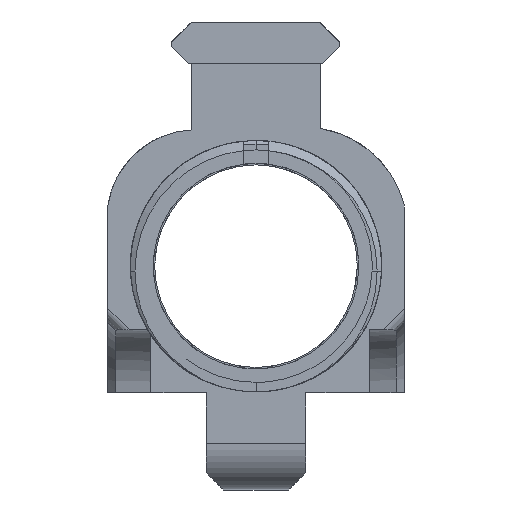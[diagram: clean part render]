
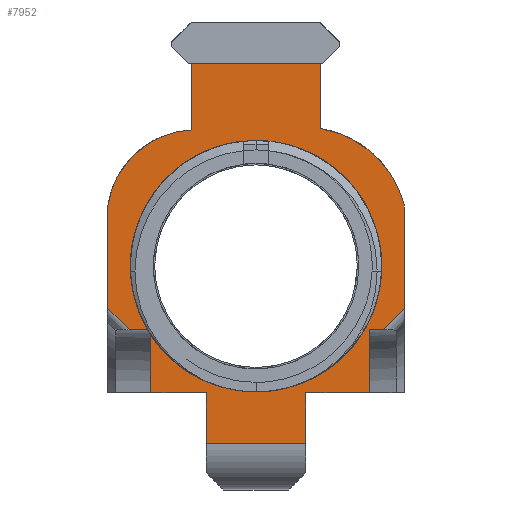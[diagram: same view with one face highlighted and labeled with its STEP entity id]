
A CAD part, front view. The second image highlights one B-rep face of the part: STEP entity #7952.
In plain terms, the highlighted planar face has unit normal (0, -1, 0).
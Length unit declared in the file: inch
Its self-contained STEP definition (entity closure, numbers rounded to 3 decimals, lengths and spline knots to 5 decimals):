
#28=FACE_BOUND('',#1369,.T.);
#355=PLANE('',#8558);
#369=CIRCLE('',#7998,0.51729);
#529=CIRCLE('',#8515,0.44384);
#537=CIRCLE('',#8557,0.58625);
#949=FACE_OUTER_BOUND('',#1368,.T.);
#1368=EDGE_LOOP('',(#7317,#7318,#7319,#7320,#7321,#7322,#7323,#7324,#7325,
#7326,#7327,#7328,#7329,#7330,#7331,#7332,#7333,#7334,#7335,#7336));
#1369=EDGE_LOOP('',(#7337));
#1472=B_SPLINE_CURVE_WITH_KNOTS('',3,(#12168,#12169,#12170,#12171),
 .UNSPECIFIED.,.F.,.F.,(4,4),(0.18081,0.55432),
 .UNSPECIFIED.);
#1555=B_SPLINE_CURVE_WITH_KNOTS('',3,(#15086,#15087,#15088,#15089),
 .UNSPECIFIED.,.F.,.F.,(4,4),(2.0691,2.45646),
 .UNSPECIFIED.);
#1620=LINE('',#11397,#2382);
#1637=LINE('',#11438,#2399);
#1769=LINE('',#12685,#2531);
#1799=LINE('',#12870,#2561);
#1881=LINE('',#13045,#2643);
#2091=LINE('',#13915,#2853);
#2271=LINE('',#14954,#3033);
#2273=LINE('',#14959,#3035);
#2275=LINE('',#14965,#3037);
#2277=LINE('',#14969,#3039);
#2283=LINE('',#14992,#3045);
#2284=LINE('',#14994,#3046);
#2290=LINE('',#15031,#3052);
#2327=LINE('',#15381,#3089);
#2358=LINE('',#16108,#3120);
#2359=LINE('',#16109,#3121);
#2382=VECTOR('',#8627,0.3937);
#2399=VECTOR('',#8654,0.3937);
#2531=VECTOR('',#8962,0.3937);
#2561=VECTOR('',#9072,0.3937);
#2643=VECTOR('',#9180,0.3937);
#2853=VECTOR('',#9658,0.494);
#3033=VECTOR('',#10202,0.3937);
#3035=VECTOR('',#10208,0.3937);
#3037=VECTOR('',#10214,0.3937);
#3039=VECTOR('',#10218,0.3937);
#3045=VECTOR('',#10234,0.3937);
#3046=VECTOR('',#10235,0.3937);
#3052=VECTOR('',#10243,0.3937);
#3089=VECTOR('',#10352,0.3937);
#3120=VECTOR('',#10473,0.3937);
#3121=VECTOR('',#10474,0.3937);
#3175=VERTEX_POINT('',#11289);
#3176=VERTEX_POINT('',#11291);
#3183=VERTEX_POINT('',#11396);
#3202=VERTEX_POINT('',#11436);
#3354=VERTEX_POINT('',#12156);
#3355=VERTEX_POINT('',#12167);
#3388=VERTEX_POINT('',#12683);
#3389=VERTEX_POINT('',#12684);
#3441=VERTEX_POINT('',#12868);
#3442=VERTEX_POINT('',#12869);
#3521=VERTEX_POINT('',#13043);
#3522=VERTEX_POINT('',#13044);
#3810=VERTEX_POINT('',#14958);
#3812=VERTEX_POINT('',#14964);
#3813=VERTEX_POINT('',#14968);
#3822=VERTEX_POINT('',#14993);
#3829=VERTEX_POINT('',#15030);
#3832=VERTEX_POINT('',#15062);
#3833=VERTEX_POINT('',#15073);
#3877=VERTEX_POINT('',#15380);
#3908=VERTEX_POINT('',#16104);
#3959=EDGE_CURVE('',#3176,#3175,#369,.T.);
#3971=EDGE_CURVE('',#3183,#3176,#1620,.T.);
#3992=EDGE_CURVE('',#3175,#3202,#1637,.F.);
#4174=EDGE_CURVE('',#3354,#3355,#1472,.T.);
#4216=EDGE_CURVE('',#3388,#3389,#1769,.F.);
#4281=EDGE_CURVE('',#3441,#3442,#1799,.T.);
#4369=EDGE_CURVE('',#3521,#3522,#1881,.F.);
#4627=EDGE_CURVE('',#3389,#3521,#2091,.T.);
#4901=EDGE_CURVE('',#3354,#3183,#2271,.T.);
#4904=EDGE_CURVE('',#3810,#3355,#2273,.T.);
#4907=EDGE_CURVE('',#3812,#3810,#2275,.T.);
#4909=EDGE_CURVE('',#3813,#3812,#2277,.T.);
#4920=EDGE_CURVE('',#3813,#3522,#2283,.T.);
#4921=EDGE_CURVE('',#3388,#3822,#2284,.T.);
#4930=EDGE_CURVE('',#3829,#3822,#2290,.T.);
#4937=EDGE_CURVE('',#3833,#3832,#1555,.T.);
#5005=EDGE_CURVE('',#3832,#3877,#2327,.T.);
#5010=EDGE_CURVE('',#3441,#3877,#529,.T.);
#5083=EDGE_CURVE('',#3908,#3908,#537,.T.);
#5084=EDGE_CURVE('',#3202,#3442,#2358,.T.);
#5085=EDGE_CURVE('',#3833,#3829,#2359,.T.);
#7317=ORIENTED_EDGE('',*,*,#5084,.T.);
#7318=ORIENTED_EDGE('',*,*,#4281,.F.);
#7319=ORIENTED_EDGE('',*,*,#5010,.T.);
#7320=ORIENTED_EDGE('',*,*,#5005,.F.);
#7321=ORIENTED_EDGE('',*,*,#4937,.F.);
#7322=ORIENTED_EDGE('',*,*,#5085,.T.);
#7323=ORIENTED_EDGE('',*,*,#4930,.T.);
#7324=ORIENTED_EDGE('',*,*,#4921,.F.);
#7325=ORIENTED_EDGE('',*,*,#4216,.T.);
#7326=ORIENTED_EDGE('',*,*,#4627,.T.);
#7327=ORIENTED_EDGE('',*,*,#4369,.T.);
#7328=ORIENTED_EDGE('',*,*,#4920,.F.);
#7329=ORIENTED_EDGE('',*,*,#4909,.T.);
#7330=ORIENTED_EDGE('',*,*,#4907,.T.);
#7331=ORIENTED_EDGE('',*,*,#4904,.T.);
#7332=ORIENTED_EDGE('',*,*,#4174,.F.);
#7333=ORIENTED_EDGE('',*,*,#4901,.T.);
#7334=ORIENTED_EDGE('',*,*,#3971,.T.);
#7335=ORIENTED_EDGE('',*,*,#3959,.T.);
#7336=ORIENTED_EDGE('',*,*,#3992,.T.);
#7337=ORIENTED_EDGE('',*,*,#5083,.T.);
#7952=ADVANCED_FACE('',(#949,#28),#355,.F.);
#7998=AXIS2_PLACEMENT_3D('',#11292,#8609,#8610);
#8515=AXIS2_PLACEMENT_3D('',#15396,#10357,#10358);
#8557=AXIS2_PLACEMENT_3D('',#16106,#10469,#10470);
#8558=AXIS2_PLACEMENT_3D('',#16107,#10471,#10472);
#8609=DIRECTION('center_axis',(0.,-1.,0.));
#8610=DIRECTION('ref_axis',(0.967,0.,0.253));
#8627=DIRECTION('',(0.,0.,1.));
#8654=DIRECTION('',(0.,0.,-1.));
#8962=DIRECTION('',(0.,0.,1.));
#9072=DIRECTION('',(0.,0.,1.));
#9180=DIRECTION('',(0.,0.,-1.));
#9658=DIRECTION('',(1.,0.,0.));
#10202=DIRECTION('',(0.,0.,1.));
#10208=DIRECTION('',(1.,0.,0.));
#10214=DIRECTION('',(0.,0.,1.));
#10218=DIRECTION('',(1.,0.,0.));
#10234=DIRECTION('',(-1.,0.,0.));
#10235=DIRECTION('',(-1.,0.,0.));
#10243=DIRECTION('',(0.,0.,-1.));
#10352=DIRECTION('',(0.,0.,1.));
#10357=DIRECTION('center_axis',(0.,-1.,0.));
#10358=DIRECTION('ref_axis',(-0.049,0.,0.999));
#10469=DIRECTION('center_axis',(0.,1.,0.));
#10470=DIRECTION('ref_axis',(1.,0.,0.));
#10471=DIRECTION('center_axis',(0.,1.,0.));
#10472=DIRECTION('ref_axis',(-1.,0.,0.));
#10473=DIRECTION('',(-1.,0.,0.));
#10474=DIRECTION('',(1.,0.,0.));
#11289=CARTESIAN_POINT('',(0.31825,-5.09153,-0.54924));
#11291=CARTESIAN_POINT('',(0.73517,-5.09153,-0.92883));
#11292=CARTESIAN_POINT('Origin',(0.23472,-5.09153,-1.05974));
#11396=CARTESIAN_POINT('',(0.73517,-5.09153,-1.02227));
#11397=CARTESIAN_POINT('',(0.73517,-5.09153,-1.02227));
#11436=CARTESIAN_POINT('',(0.31825,-5.09153,-0.22581));
#11438=CARTESIAN_POINT('',(0.31825,-5.09153,-1.26173));
#12156=CARTESIAN_POINT('',(0.73517,-5.09153,-1.44277));
#12167=CARTESIAN_POINT('',(0.63217,-5.09153,-1.54771));
#12168=CARTESIAN_POINT('Ctrl Pts',(0.73517,-5.09153,
-1.44277));
#12169=CARTESIAN_POINT('Ctrl Pts',(0.70077,-5.09153,-1.47768));
#12170=CARTESIAN_POINT('Ctrl Pts',(0.66642,-5.09153,
-1.51265));
#12171=CARTESIAN_POINT('Ctrl Pts',(0.63217,-5.09153,
-1.54771));
#12683=CARTESIAN_POINT('',(-0.24725,-5.09153,-1.86173));
#12684=CARTESIAN_POINT('',(-0.24725,-5.09153,-2.11173));
#12685=CARTESIAN_POINT('',(-0.24725,-5.09153,-2.18471));
#12868=CARTESIAN_POINT('',(-0.31875,-5.09153,-0.5563));
#12869=CARTESIAN_POINT('',(-0.31875,-5.09153,-0.22581));
#12870=CARTESIAN_POINT('',(-0.31875,-5.09153,-1.39849));
#13043=CARTESIAN_POINT('',(0.24675,-5.09153,-2.11173));
#13044=CARTESIAN_POINT('',(0.24675,-5.09153,-1.86173));
#13045=CARTESIAN_POINT('',(0.24675,-5.09153,-1.98673));
#13915=CARTESIAN_POINT('',(-0.24725,-5.09153,-2.11173));
#14954=CARTESIAN_POINT('',(0.73517,-5.09153,-1.86173));
#14958=CARTESIAN_POINT('',(0.5625,-5.09153,-1.54771));
#14959=CARTESIAN_POINT('',(0.73517,-5.09153,-1.54771));
#14964=CARTESIAN_POINT('',(0.5625,-5.09153,-1.86173));
#14965=CARTESIAN_POINT('',(0.5625,-5.09153,-1.77686));
#14968=CARTESIAN_POINT('',(0.43725,-5.09153,-1.86173));
#14969=CARTESIAN_POINT('',(0.43725,-5.09153,-1.86173));
#14992=CARTESIAN_POINT('',(-0.58511,-5.09153,-1.86173));
#14993=CARTESIAN_POINT('',(-0.522,-5.09153,-1.86173));
#14994=CARTESIAN_POINT('',(-0.29291,-5.09153,-1.86173));
#15030=CARTESIAN_POINT('',(-0.522,-5.09153,-1.54848));
#15031=CARTESIAN_POINT('',(-0.522,-5.09153,-1.75467));
#15062=CARTESIAN_POINT('',(-0.73605,-5.09153,-1.44027));
#15073=CARTESIAN_POINT('',(-0.62859,-5.09153,-1.54848));
#15086=CARTESIAN_POINT('Ctrl Pts',(-0.62859,-5.09153,
-1.54848));
#15087=CARTESIAN_POINT('Ctrl Pts',(-0.66437,-5.09153,
-1.51237));
#15088=CARTESIAN_POINT('Ctrl Pts',(-0.7002,-5.09153,
-1.47631));
#15089=CARTESIAN_POINT('Ctrl Pts',(-0.73605,-5.09153,
-1.44027));
#15380=CARTESIAN_POINT('',(-0.73605,-5.09153,-0.93348));
#15381=CARTESIAN_POINT('',(-0.73605,-5.09153,-1.86173));
#15396=CARTESIAN_POINT('Origin',(-0.29716,-5.09153,-0.99962));
#16104=CARTESIAN_POINT('',(-0.5865,-5.09153,-1.23273));
#16106=CARTESIAN_POINT('Origin',(-0.00025,-5.09153,
-1.23273));
#16107=CARTESIAN_POINT('Origin',(-0.60748,-5.09153,-2.11173));
#16108=CARTESIAN_POINT('',(-0.47162,-5.09153,-0.22581));
#16109=CARTESIAN_POINT('',(-0.73605,-5.09153,-1.54848));
